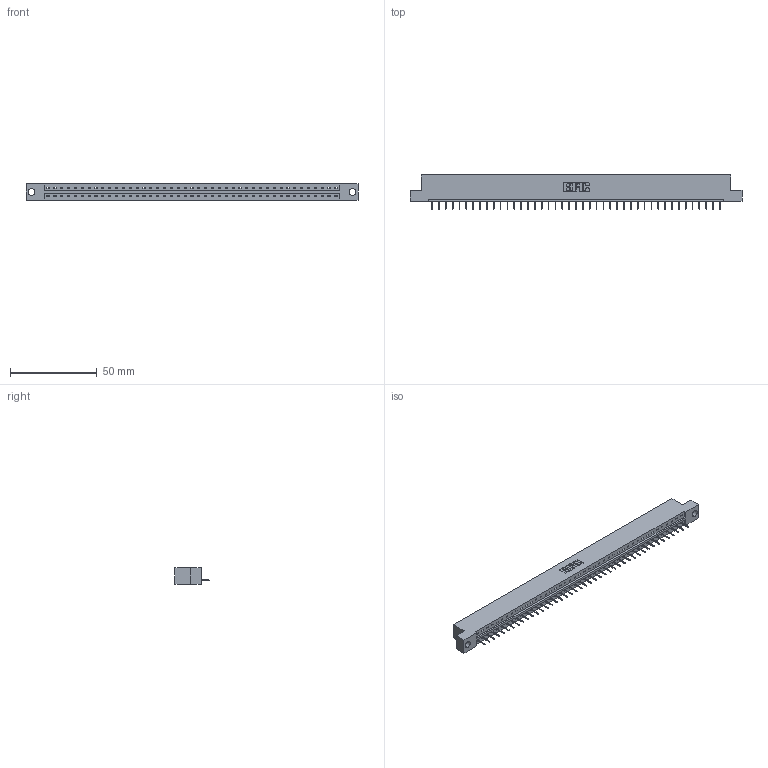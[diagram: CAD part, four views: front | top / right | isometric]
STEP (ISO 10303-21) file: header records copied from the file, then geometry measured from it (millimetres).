
FILE_DESCRIPTION (( 'STEP AP203' ), '1' );
FILE_NAME ('833-043-524-104.STEP', '2020-06-03T23:38:25', ( '' ), ( '' ), 'SwSTEP 2.0', 'SolidWorks 2020', '' );
FILE_SCHEMA (( 'CONFIG_CONTROL_DESIGN' ));
Length unit declared in the file: inch
Products named in the file (3): 833 Part_Flush - .156 Dia - TH; 833-043-524-104; 345-292-001_345-293-124
Assembly tree (44 placements, depth 2):
  833-043-524-104
    833 Part_Flush - .156 Dia - TH
    345-292-001_345-293-124  x43
Bounding box: 191.92 x 19.69 x 9.4 mm (x, y, z)
Volume: 19063.7 mm3; surface area: 19844.8 mm2
Topology: 44 solids, 44 shells, 2780 faces, 8051 edges, 5194 vertices
Faces by surface type: plane 2134, cylinder 646
Entity records: 26235 total; most frequent: CARTESIAN_POINT 4531, ORIENTED_EDGE 4510, DIRECTION 3821, EDGE_CURVE 2255, LINE 2131, VECTOR 2131, VERTEX_POINT 1498, AXIS2_PLACEMENT_3D 845
